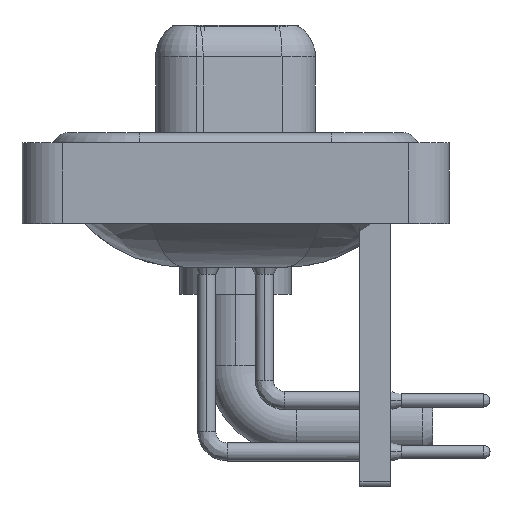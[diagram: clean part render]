
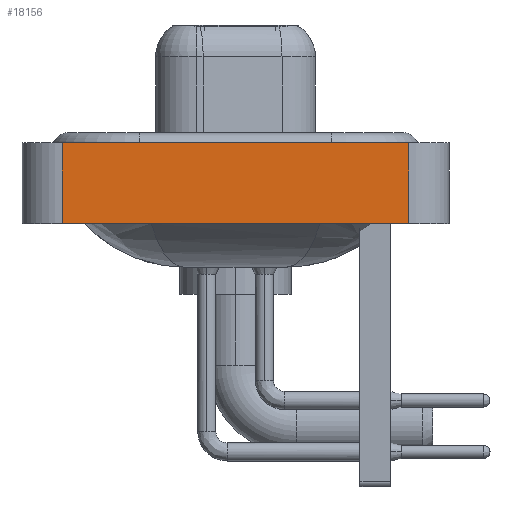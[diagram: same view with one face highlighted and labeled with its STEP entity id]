
A CAD part, left-side view. The second image highlights one B-rep face of the part: STEP entity #18156.
In plain terms, the highlighted planar face has unit normal (-1, 0, 0).
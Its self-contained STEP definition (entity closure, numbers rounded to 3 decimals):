
#41 = LINE ( 'NONE', #25320, #23496 ) ;
#117 = PLANE ( 'NONE',  #25468 ) ;
#259 = DIRECTION ( 'NONE',  ( -1., 0., 0. ) ) ;
#1169 = EDGE_CURVE ( 'NONE', #14016, #23230, #24956, .T. ) ;
#1488 = CARTESIAN_POINT ( 'NONE',  ( -7.35, -8.55, -3.6 ) ) ;
#2877 = LINE ( 'NONE', #8654, #15355 ) ;
#3631 = ORIENTED_EDGE ( 'NONE', *, *, #17165, .T. ) ;
#3805 = DIRECTION ( 'NONE',  ( 0., 0., 1. ) ) ;
#5191 = EDGE_LOOP ( 'NONE', ( #27248, #25702, #25502, #3631 ) ) ;
#5294 = CARTESIAN_POINT ( 'NONE',  ( -7.35, 8.55, 0.4 ) ) ;
#7942 = VERTEX_POINT ( 'NONE', #5294 ) ;
#7945 = VECTOR ( 'NONE', #20263, 1000. ) ;
#8650 = DIRECTION ( 'NONE',  ( 0., 0., 1. ) ) ;
#8654 = CARTESIAN_POINT ( 'NONE',  ( -7.35, -8.55, 0.4 ) ) ;
#10656 = DIRECTION ( 'NONE',  ( 0., -1., 0. ) ) ;
#11505 = VECTOR ( 'NONE', #3805, 1000. ) ;
#12424 = EDGE_CURVE ( 'NONE', #7942, #23230, #2877, .T. ) ;
#12660 = FACE_OUTER_BOUND ( 'NONE', #5191, .T. ) ;
#14016 = VERTEX_POINT ( 'NONE', #1488 ) ;
#14040 = LINE ( 'NONE', #24678, #7945 ) ;
#14129 = EDGE_CURVE ( 'NONE', #19510, #7942, #14040, .T. ) ;
#15355 = VECTOR ( 'NONE', #17101, 1000. ) ;
#16965 = CARTESIAN_POINT ( 'NONE',  ( -7.35, -8.55, -3.6 ) ) ;
#17101 = DIRECTION ( 'NONE',  ( 0., -1., 0. ) ) ;
#17165 = EDGE_CURVE ( 'NONE', #19510, #14016, #41, .T. ) ;
#18156 = ADVANCED_FACE ( 'NONE', ( #12660 ), #117, .T. ) ;
#18407 = CARTESIAN_POINT ( 'NONE',  ( -7.35, -8.55, 0.4 ) ) ;
#19510 = VERTEX_POINT ( 'NONE', #24105 ) ;
#20263 = DIRECTION ( 'NONE',  ( 0., 0., 1. ) ) ;
#22743 = CARTESIAN_POINT ( 'NONE',  ( -7.35, -8.55, -3.6 ) ) ;
#23230 = VERTEX_POINT ( 'NONE', #18407 ) ;
#23496 = VECTOR ( 'NONE', #10656, 1000. ) ;
#24105 = CARTESIAN_POINT ( 'NONE',  ( -7.35, 8.55, -3.6 ) ) ;
#24678 = CARTESIAN_POINT ( 'NONE',  ( -7.35, 8.55, -3.6 ) ) ;
#24956 = LINE ( 'NONE', #22743, #11505 ) ;
#25320 = CARTESIAN_POINT ( 'NONE',  ( -7.35, -8.55, -3.6 ) ) ;
#25468 = AXIS2_PLACEMENT_3D ( 'NONE', #16965, #259, #8650 ) ;
#25502 = ORIENTED_EDGE ( 'NONE', *, *, #14129, .F. ) ;
#25702 = ORIENTED_EDGE ( 'NONE', *, *, #12424, .F. ) ;
#27248 = ORIENTED_EDGE ( 'NONE', *, *, #1169, .T. ) ;
